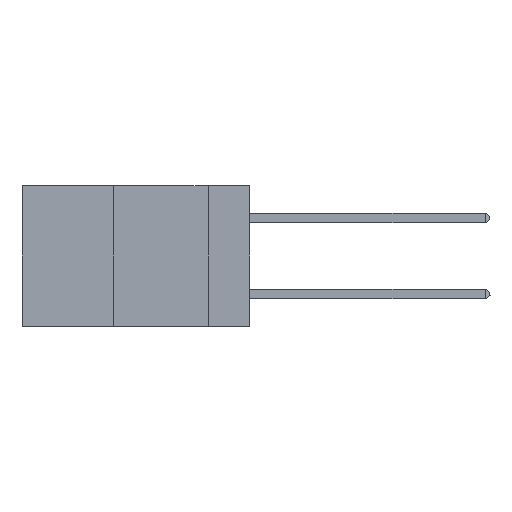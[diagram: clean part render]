
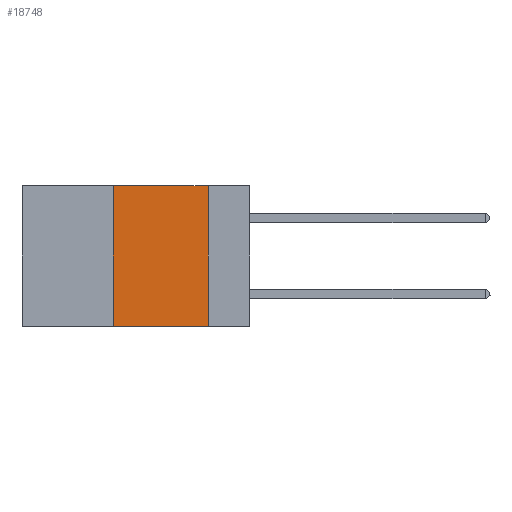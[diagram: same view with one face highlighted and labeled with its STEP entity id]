
A CAD part, left-side view. The second image highlights one B-rep face of the part: STEP entity #18748.
In plain terms, the highlighted planar face has unit normal (-1, 0, 0).
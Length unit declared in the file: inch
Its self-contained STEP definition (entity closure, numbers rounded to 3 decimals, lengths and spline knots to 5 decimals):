
#676 = CARTESIAN_POINT ( 'NONE',  ( 0., 0.11, -0.37 ) ) ;
#829 = FACE_OUTER_BOUND ( 'NONE', #8321, .T. ) ;
#1483 = DIRECTION ( 'NONE',  ( 0., -1., 0. ) ) ;
#1949 = VECTOR ( 'NONE', #5955, 39.37008 ) ;
#2953 = DIRECTION ( 'NONE',  ( 0., 0., -1. ) ) ;
#2956 = LINE ( 'NONE', #14019, #4222 ) ;
#3101 = ORIENTED_EDGE ( 'NONE', *, *, #7569, .F. ) ;
#3238 = LINE ( 'NONE', #14090, #1949 ) ;
#3475 = EDGE_CURVE ( 'NONE', #14434, #18686, #3238, .T. ) ;
#4222 = VECTOR ( 'NONE', #1483, 39.37008 ) ;
#4819 = CARTESIAN_POINT ( 'NONE',  ( 0., 0.6, 0. ) ) ;
#5955 = DIRECTION ( 'NONE',  ( 0., -1., 0. ) ) ;
#6651 = LINE ( 'NONE', #19648, #26588 ) ;
#6883 = CARTESIAN_POINT ( 'NONE',  ( 0., 0.36, 0. ) ) ;
#7009 = AXIS2_PLACEMENT_3D ( 'NONE', #4819, #13206, #2953 ) ;
#7238 = PLANE ( 'NONE',  #7009 ) ;
#7569 = EDGE_CURVE ( 'NONE', #11795, #16474, #2956, .T. ) ;
#7817 = DIRECTION ( 'NONE',  ( 0., 0., 1. ) ) ;
#8321 = EDGE_LOOP ( 'NONE', ( #14561, #3101, #12363, #13651 ) ) ;
#11795 = VERTEX_POINT ( 'NONE', #6883 ) ;
#12098 = LINE ( 'NONE', #22136, #17882 ) ;
#12363 = ORIENTED_EDGE ( 'NONE', *, *, #21095, .F. ) ;
#13206 = DIRECTION ( 'NONE',  ( 1., 0., 0. ) ) ;
#13651 = ORIENTED_EDGE ( 'NONE', *, *, #3475, .T. ) ;
#14019 = CARTESIAN_POINT ( 'NONE',  ( 0., 0.6, 0. ) ) ;
#14090 = CARTESIAN_POINT ( 'NONE',  ( 0., 0.6, -0.37 ) ) ;
#14434 = VERTEX_POINT ( 'NONE', #25733 ) ;
#14561 = ORIENTED_EDGE ( 'NONE', *, *, #21605, .F. ) ;
#16474 = VERTEX_POINT ( 'NONE', #23984 ) ;
#17882 = VECTOR ( 'NONE', #7817, 39.37008 ) ;
#18686 = VERTEX_POINT ( 'NONE', #676 ) ;
#18748 = ADVANCED_FACE ( 'NONE', ( #829 ), #7238, .F. ) ;
#19648 = CARTESIAN_POINT ( 'NONE',  ( 0., 0.11, 0. ) ) ;
#21095 = EDGE_CURVE ( 'NONE', #14434, #11795, #12098, .T. ) ;
#21605 = EDGE_CURVE ( 'NONE', #16474, #18686, #6651, .T. ) ;
#22136 = CARTESIAN_POINT ( 'NONE',  ( 0., 0.36, 0. ) ) ;
#23984 = CARTESIAN_POINT ( 'NONE',  ( 0., 0.11, 0. ) ) ;
#25733 = CARTESIAN_POINT ( 'NONE',  ( 0., 0.36, -0.37 ) ) ;
#25780 = DIRECTION ( 'NONE',  ( 0., 0., -1. ) ) ;
#26588 = VECTOR ( 'NONE', #25780, 39.37008 ) ;
